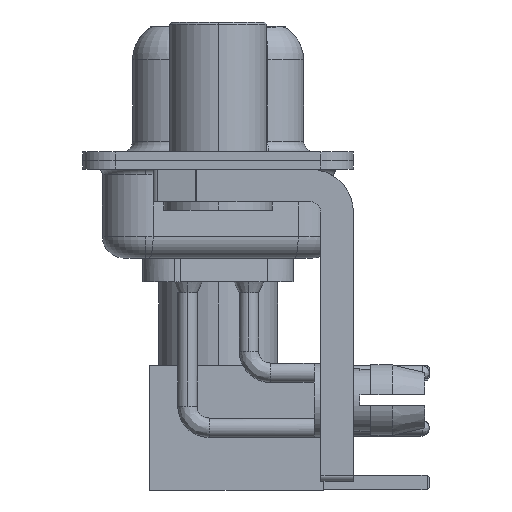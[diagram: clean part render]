
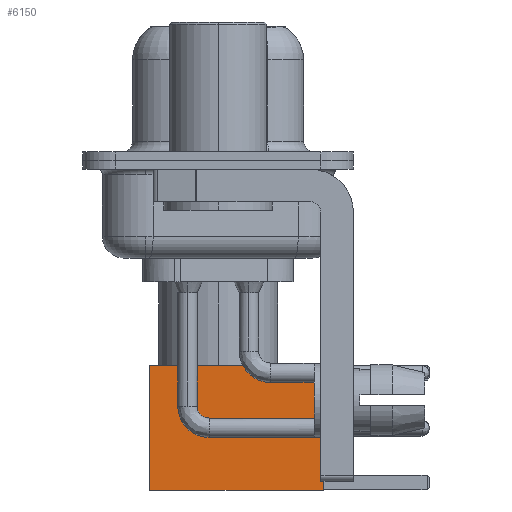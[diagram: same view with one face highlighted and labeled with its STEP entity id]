
A CAD part, left-side view. The second image highlights one B-rep face of the part: STEP entity #6150.
In plain terms, the highlighted face is planar.
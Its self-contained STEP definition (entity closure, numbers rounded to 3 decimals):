
#1377 = ORIENTED_EDGE ( 'NONE', *, *, #23246, .F. ) ;
#1712 = DIRECTION ( 'NONE',  ( 0., 0., 1. ) ) ;
#2269 = EDGE_CURVE ( 'NONE', #17534, #3442, #3835, .T. ) ;
#2676 = PLANE ( 'NONE',  #17109 ) ;
#3333 = CARTESIAN_POINT ( 'NONE',  ( 2.875, 2.875, 0. ) ) ;
#3424 = DIRECTION ( 'NONE',  ( -1., 0., 0. ) ) ;
#3442 = VERTEX_POINT ( 'NONE', #5150 ) ;
#3835 = LINE ( 'NONE', #12269, #14184 ) ;
#4917 = CARTESIAN_POINT ( 'NONE',  ( 0., 2.875, 0. ) ) ;
#5065 = VERTEX_POINT ( 'NONE', #13226 ) ;
#5150 = CARTESIAN_POINT ( 'NONE',  ( -2.875, 2.875, 8. ) ) ;
#5214 = CARTESIAN_POINT ( 'NONE',  ( 2.875, 2.875, 0. ) ) ;
#6040 = ORIENTED_EDGE ( 'NONE', *, *, #11598, .T. ) ;
#6150 = ADVANCED_FACE ( 'NONE', ( #7104 ), #2676, .T. ) ;
#6306 = EDGE_LOOP ( 'NONE', ( #23571, #6040, #1377, #22970 ) ) ;
#7104 = FACE_OUTER_BOUND ( 'NONE', #6306, .T. ) ;
#7489 = VECTOR ( 'NONE', #3424, 1000. ) ;
#8224 = VECTOR ( 'NONE', #11366, 1000. ) ;
#9492 = LINE ( 'NONE', #5214, #8224 ) ;
#11366 = DIRECTION ( 'NONE',  ( 0., 0., -1. ) ) ;
#11520 = DIRECTION ( 'NONE',  ( 0., 1., 0. ) ) ;
#11598 = EDGE_CURVE ( 'NONE', #5065, #22641, #17623, .T. ) ;
#11867 = CARTESIAN_POINT ( 'NONE',  ( 2.875, 2.875, 8. ) ) ;
#12269 = CARTESIAN_POINT ( 'NONE',  ( 0., 2.875, 8. ) ) ;
#13226 = CARTESIAN_POINT ( 'NONE',  ( 2.875, 2.875, 0. ) ) ;
#13561 = LINE ( 'NONE', #25618, #17304 ) ;
#14184 = VECTOR ( 'NONE', #24733, 1000. ) ;
#15445 = DIRECTION ( 'NONE',  ( 0., 0., -1. ) ) ;
#17109 = AXIS2_PLACEMENT_3D ( 'NONE', #3333, #11520, #1712 ) ;
#17304 = VECTOR ( 'NONE', #15445, 1000. ) ;
#17534 = VERTEX_POINT ( 'NONE', #11867 ) ;
#17623 = LINE ( 'NONE', #4917, #7489 ) ;
#22024 = EDGE_CURVE ( 'NONE', #17534, #5065, #9492, .T. ) ;
#22641 = VERTEX_POINT ( 'NONE', #24002 ) ;
#22970 = ORIENTED_EDGE ( 'NONE', *, *, #2269, .F. ) ;
#23246 = EDGE_CURVE ( 'NONE', #3442, #22641, #13561, .T. ) ;
#23571 = ORIENTED_EDGE ( 'NONE', *, *, #22024, .T. ) ;
#24002 = CARTESIAN_POINT ( 'NONE',  ( -2.875, 2.875, 0. ) ) ;
#24733 = DIRECTION ( 'NONE',  ( -1., 0., 0. ) ) ;
#25618 = CARTESIAN_POINT ( 'NONE',  ( -2.875, 2.875, 0. ) ) ;
